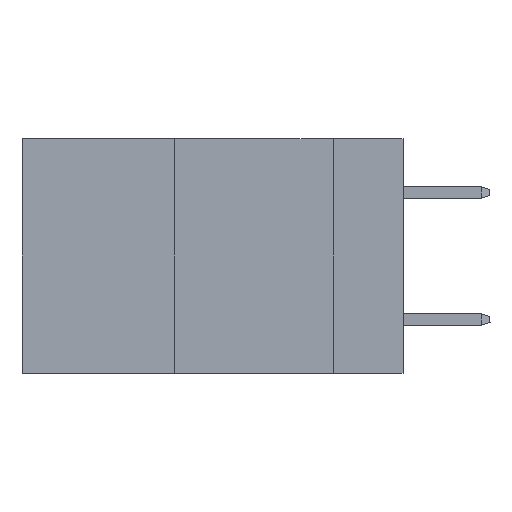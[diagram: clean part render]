
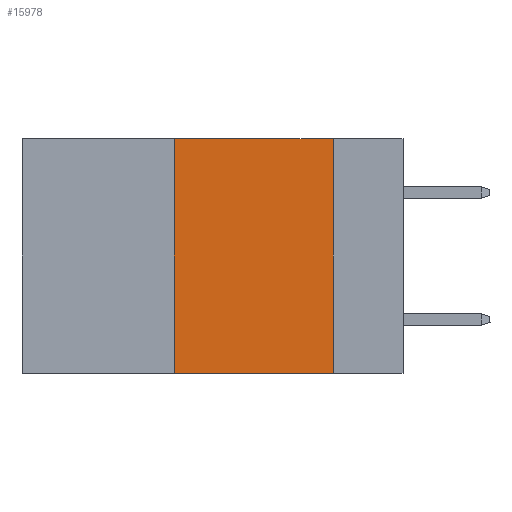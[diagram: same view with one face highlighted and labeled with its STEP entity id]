
A CAD part, left-side view. The second image highlights one B-rep face of the part: STEP entity #15978.
In plain terms, the highlighted planar face has unit normal (-1, 0, 0).
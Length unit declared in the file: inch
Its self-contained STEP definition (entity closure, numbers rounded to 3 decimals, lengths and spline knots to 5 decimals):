
#2384 = VERTEX_POINT ( 'NONE', #5815 ) ;
#2458 = CARTESIAN_POINT ( 'NONE',  ( 0., 0.11, 0. ) ) ;
#3538 = VECTOR ( 'NONE', #22156, 39.37008 ) ;
#5815 = CARTESIAN_POINT ( 'NONE',  ( 0., 0.36, -0.37 ) ) ;
#6336 = VERTEX_POINT ( 'NONE', #13777 ) ;
#6579 = DIRECTION ( 'NONE',  ( 1., 0., 0. ) ) ;
#6593 = ORIENTED_EDGE ( 'NONE', *, *, #19838, .T. ) ;
#7884 = DIRECTION ( 'NONE',  ( 0., 0., 1. ) ) ;
#8012 = EDGE_CURVE ( 'NONE', #22917, #6336, #19523, .T. ) ;
#8615 = CARTESIAN_POINT ( 'NONE',  ( 0., 0.11, 0. ) ) ;
#8982 = EDGE_CURVE ( 'NONE', #21383, #22917, #18049, .T. ) ;
#9653 = CARTESIAN_POINT ( 'NONE',  ( 0., 0.6, -0.37 ) ) ;
#9971 = ORIENTED_EDGE ( 'NONE', *, *, #22816, .F. ) ;
#10689 = DIRECTION ( 'NONE',  ( 0., 0., -1. ) ) ;
#11121 = VECTOR ( 'NONE', #17651, 39.37008 ) ;
#11794 = ORIENTED_EDGE ( 'NONE', *, *, #8982, .F. ) ;
#11894 = DIRECTION ( 'NONE',  ( 0., -1., 0. ) ) ;
#11996 = CARTESIAN_POINT ( 'NONE',  ( 0., 0.36, 0. ) ) ;
#12547 = PLANE ( 'NONE',  #13082 ) ;
#13082 = AXIS2_PLACEMENT_3D ( 'NONE', #20140, #6579, #10689 ) ;
#13777 = CARTESIAN_POINT ( 'NONE',  ( 0., 0.11, -0.37 ) ) ;
#14435 = VECTOR ( 'NONE', #11894, 39.37008 ) ;
#14564 = CARTESIAN_POINT ( 'NONE',  ( 0., 0.6, 0. ) ) ;
#15978 = ADVANCED_FACE ( 'NONE', ( #23643 ), #12547, .F. ) ;
#17550 = EDGE_LOOP ( 'NONE', ( #23361, #11794, #9971, #6593 ) ) ;
#17651 = DIRECTION ( 'NONE',  ( 0., 0., -1. ) ) ;
#17719 = LINE ( 'NONE', #9653, #14435 ) ;
#18049 = LINE ( 'NONE', #14564, #3538 ) ;
#19523 = LINE ( 'NONE', #2458, #11121 ) ;
#19838 = EDGE_CURVE ( 'NONE', #2384, #6336, #17719, .T. ) ;
#20140 = CARTESIAN_POINT ( 'NONE',  ( 0., 0.6, 0. ) ) ;
#20830 = CARTESIAN_POINT ( 'NONE',  ( 0., 0.36, 0. ) ) ;
#21383 = VERTEX_POINT ( 'NONE', #20830 ) ;
#21563 = LINE ( 'NONE', #11996, #23895 ) ;
#22156 = DIRECTION ( 'NONE',  ( 0., -1., 0. ) ) ;
#22816 = EDGE_CURVE ( 'NONE', #2384, #21383, #21563, .T. ) ;
#22917 = VERTEX_POINT ( 'NONE', #8615 ) ;
#23361 = ORIENTED_EDGE ( 'NONE', *, *, #8012, .F. ) ;
#23643 = FACE_OUTER_BOUND ( 'NONE', #17550, .T. ) ;
#23895 = VECTOR ( 'NONE', #7884, 39.37008 ) ;
